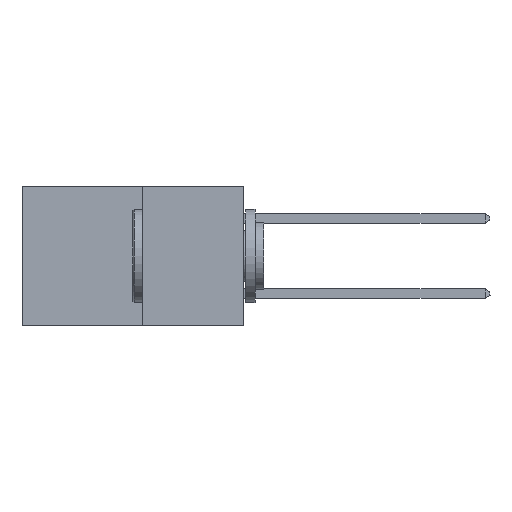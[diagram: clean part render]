
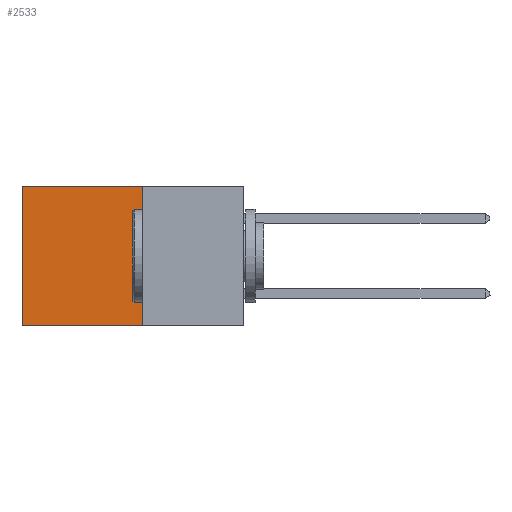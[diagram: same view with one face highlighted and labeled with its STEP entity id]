
A CAD part, left-side view. The second image highlights one B-rep face of the part: STEP entity #2533.
In plain terms, the highlighted planar face has unit normal (-1, 0, 0).
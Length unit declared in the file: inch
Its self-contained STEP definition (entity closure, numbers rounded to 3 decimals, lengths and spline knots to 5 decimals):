
#1054 = FACE_OUTER_BOUND ( 'NONE', #32469, .T. ) ;
#1874 = CARTESIAN_POINT ( 'NONE',  ( 0.277, 0.27, 0. ) ) ;
#2533 = ADVANCED_FACE ( 'NONE', ( #1054 ), #24718, .F. ) ;
#3578 = VECTOR ( 'NONE', #8386, 39.37008 ) ;
#4672 = CARTESIAN_POINT ( 'NONE',  ( 0.277, 0.27, -0.37 ) ) ;
#5678 = CARTESIAN_POINT ( 'NONE',  ( 0.277, 0.27, -0.37 ) ) ;
#5880 = EDGE_CURVE ( 'NONE', #28401, #33225, #15199, .T. ) ;
#6864 = DIRECTION ( 'NONE',  ( 0., 0., -1. ) ) ;
#7185 = VECTOR ( 'NONE', #21459, 39.37008 ) ;
#7294 = VECTOR ( 'NONE', #6864, 39.37008 ) ;
#7346 = LINE ( 'NONE', #27165, #14527 ) ;
#8386 = DIRECTION ( 'NONE',  ( 0., 1., 0. ) ) ;
#8420 = ORIENTED_EDGE ( 'NONE', *, *, #5880, .T. ) ;
#10363 = CARTESIAN_POINT ( 'NONE',  ( 0.277, 0.59, 0. ) ) ;
#11367 = DIRECTION ( 'NONE',  ( 1., 0., 0. ) ) ;
#11801 = VERTEX_POINT ( 'NONE', #16576 ) ;
#14527 = VECTOR ( 'NONE', #32550, 39.37008 ) ;
#15199 = LINE ( 'NONE', #34748, #7185 ) ;
#16576 = CARTESIAN_POINT ( 'NONE',  ( 0.277, 0.59, -0.37 ) ) ;
#16950 = EDGE_CURVE ( 'NONE', #33225, #11801, #7346, .T. ) ;
#18188 = AXIS2_PLACEMENT_3D ( 'NONE', #27382, #11367, #30064 ) ;
#21459 = DIRECTION ( 'NONE',  ( 0., 1., 0. ) ) ;
#22316 = EDGE_CURVE ( 'NONE', #28401, #27537, #29501, .T. ) ;
#24567 = ORIENTED_EDGE ( 'NONE', *, *, #16950, .T. ) ;
#24718 = PLANE ( 'NONE',  #18188 ) ;
#25025 = LINE ( 'NONE', #5678, #3578 ) ;
#25627 = CARTESIAN_POINT ( 'NONE',  ( 0.277, 0.27, -0.37 ) ) ;
#27165 = CARTESIAN_POINT ( 'NONE',  ( 0.277, 0.59, -0.37 ) ) ;
#27382 = CARTESIAN_POINT ( 'NONE',  ( 0.277, 0.27, -0.37 ) ) ;
#27537 = VERTEX_POINT ( 'NONE', #4672 ) ;
#27962 = ORIENTED_EDGE ( 'NONE', *, *, #22316, .F. ) ;
#28401 = VERTEX_POINT ( 'NONE', #1874 ) ;
#29501 = LINE ( 'NONE', #25627, #7294 ) ;
#30064 = DIRECTION ( 'NONE',  ( 0., 0., -1. ) ) ;
#32469 = EDGE_LOOP ( 'NONE', ( #24567, #33045, #27962, #8420 ) ) ;
#32550 = DIRECTION ( 'NONE',  ( 0., 0., -1. ) ) ;
#32674 = EDGE_CURVE ( 'NONE', #27537, #11801, #25025, .T. ) ;
#33045 = ORIENTED_EDGE ( 'NONE', *, *, #32674, .F. ) ;
#33225 = VERTEX_POINT ( 'NONE', #10363 ) ;
#34748 = CARTESIAN_POINT ( 'NONE',  ( 0.277, 0.27, 0. ) ) ;
